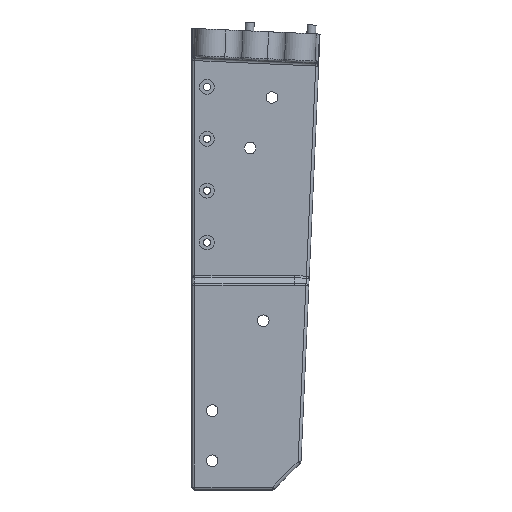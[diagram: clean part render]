
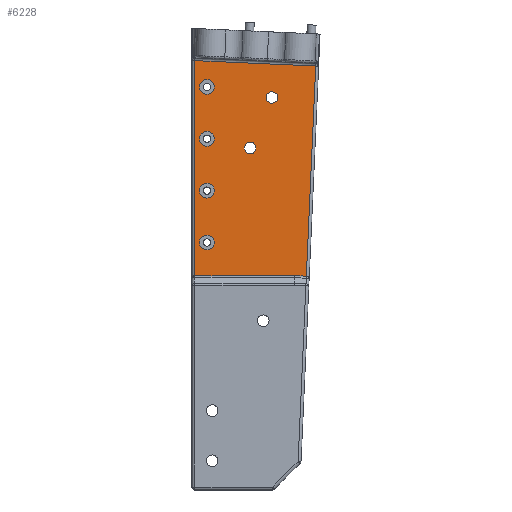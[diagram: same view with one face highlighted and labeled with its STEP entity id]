
A CAD part, left-side view. The second image highlights one B-rep face of the part: STEP entity #6228.
In plain terms, the highlighted planar face has unit normal (-1, 0, 0).
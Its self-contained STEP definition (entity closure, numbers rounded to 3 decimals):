
#161=ELLIPSE('',#6764,2.83,2.);
#335=LINE('',#9959,#885);
#356=LINE('',#10603,#906);
#358=LINE('',#10630,#908);
#368=LINE('',#10674,#918);
#369=LINE('',#10676,#919);
#885=VECTOR('',#7695,10.);
#906=VECTOR('',#7892,10.);
#908=VECTOR('',#7904,10.);
#918=VECTOR('',#7932,10.);
#919=VECTOR('',#7935,10.);
#1436=FACE_BOUND('',#2027,.T.);
#1437=FACE_BOUND('',#2028,.T.);
#1438=FACE_BOUND('',#2029,.T.);
#1439=FACE_BOUND('',#2030,.T.);
#1440=FACE_BOUND('',#2031,.T.);
#1441=FACE_BOUND('',#2032,.T.);
#1622=FACE_OUTER_BOUND('',#2026,.T.);
#2026=EDGE_LOOP('',(#4883,#4884,#4885,#4886,#4887,#4888));
#2027=EDGE_LOOP('',(#4889,#4890));
#2028=EDGE_LOOP('',(#4891,#4892));
#2029=EDGE_LOOP('',(#4893,#4894));
#2030=EDGE_LOOP('',(#4895,#4896));
#2031=EDGE_LOOP('',(#4897,#4898));
#2032=EDGE_LOOP('',(#4899));
#2284=CIRCLE('',#6493,2.54);
#2285=CIRCLE('',#6494,2.54);
#2289=CIRCLE('',#6500,2.54);
#2290=CIRCLE('',#6501,2.54);
#2294=CIRCLE('',#6507,2.54);
#2295=CIRCLE('',#6508,2.54);
#2299=CIRCLE('',#6514,2.54);
#2300=CIRCLE('',#6515,2.54);
#2474=CIRCLE('',#6821,2.);
#2475=CIRCLE('',#6822,2.);
#2476=CIRCLE('',#6823,2.);
#2621=VERTEX_POINT('',#9115);
#2622=VERTEX_POINT('',#9117);
#2626=VERTEX_POINT('',#9128);
#2627=VERTEX_POINT('',#9130);
#2631=VERTEX_POINT('',#9141);
#2632=VERTEX_POINT('',#9143);
#2636=VERTEX_POINT('',#9154);
#2637=VERTEX_POINT('',#9156);
#2790=VERTEX_POINT('',#9945);
#2794=VERTEX_POINT('',#9957);
#2872=VERTEX_POINT('',#10594);
#2875=VERTEX_POINT('',#10601);
#2877=VERTEX_POINT('',#10622);
#2879=VERTEX_POINT('',#10628);
#2905=VERTEX_POINT('',#10844);
#2906=VERTEX_POINT('',#10845);
#2907=VERTEX_POINT('',#10848);
#3219=EDGE_CURVE('',#2622,#2621,#2284,.T.);
#3220=EDGE_CURVE('',#2621,#2622,#2285,.T.);
#3225=EDGE_CURVE('',#2627,#2626,#2289,.T.);
#3226=EDGE_CURVE('',#2626,#2627,#2290,.T.);
#3231=EDGE_CURVE('',#2632,#2631,#2294,.T.);
#3232=EDGE_CURVE('',#2631,#2632,#2295,.T.);
#3237=EDGE_CURVE('',#2637,#2636,#2299,.T.);
#3238=EDGE_CURVE('',#2636,#2637,#2300,.T.);
#3453=EDGE_CURVE('',#2794,#2790,#335,.T.);
#3564=EDGE_CURVE('',#2875,#2872,#356,.T.);
#3567=EDGE_CURVE('',#2877,#2875,#161,.T.);
#3570=EDGE_CURVE('',#2879,#2877,#358,.T.);
#3584=EDGE_CURVE('',#2872,#2794,#368,.T.);
#3585=EDGE_CURVE('',#2790,#2879,#369,.T.);
#3637=EDGE_CURVE('',#2905,#2906,#2474,.T.);
#3638=EDGE_CURVE('',#2906,#2905,#2475,.T.);
#3639=EDGE_CURVE('',#2907,#2907,#2476,.T.);
#4883=ORIENTED_EDGE('',*,*,#3453,.F.);
#4884=ORIENTED_EDGE('',*,*,#3584,.F.);
#4885=ORIENTED_EDGE('',*,*,#3564,.F.);
#4886=ORIENTED_EDGE('',*,*,#3567,.F.);
#4887=ORIENTED_EDGE('',*,*,#3570,.F.);
#4888=ORIENTED_EDGE('',*,*,#3585,.F.);
#4889=ORIENTED_EDGE('',*,*,#3219,.T.);
#4890=ORIENTED_EDGE('',*,*,#3220,.T.);
#4891=ORIENTED_EDGE('',*,*,#3225,.T.);
#4892=ORIENTED_EDGE('',*,*,#3226,.T.);
#4893=ORIENTED_EDGE('',*,*,#3231,.T.);
#4894=ORIENTED_EDGE('',*,*,#3232,.T.);
#4895=ORIENTED_EDGE('',*,*,#3237,.T.);
#4896=ORIENTED_EDGE('',*,*,#3238,.T.);
#4897=ORIENTED_EDGE('',*,*,#3637,.T.);
#4898=ORIENTED_EDGE('',*,*,#3638,.T.);
#4899=ORIENTED_EDGE('',*,*,#3639,.T.);
#5942=PLANE('',#6820);
#6228=ADVANCED_FACE('',(#1622,#1436,#1437,#1438,#1439,#1440,#1441),#5942,
 .F.);
#6493=AXIS2_PLACEMENT_3D('',#9118,#7232,#7233);
#6494=AXIS2_PLACEMENT_3D('',#9119,#7234,#7235);
#6500=AXIS2_PLACEMENT_3D('',#9131,#7247,#7248);
#6501=AXIS2_PLACEMENT_3D('',#9132,#7249,#7250);
#6507=AXIS2_PLACEMENT_3D('',#9144,#7262,#7263);
#6508=AXIS2_PLACEMENT_3D('',#9145,#7264,#7265);
#6514=AXIS2_PLACEMENT_3D('',#9157,#7277,#7278);
#6515=AXIS2_PLACEMENT_3D('',#9158,#7279,#7280);
#6764=AXIS2_PLACEMENT_3D('',#10624,#7896,#7897);
#6820=AXIS2_PLACEMENT_3D('',#10843,#8059,#8060);
#6821=AXIS2_PLACEMENT_3D('',#10846,#8061,#8062);
#6822=AXIS2_PLACEMENT_3D('',#10847,#8063,#8064);
#6823=AXIS2_PLACEMENT_3D('',#10849,#8065,#8066);
#7232=DIRECTION('center_axis',(1.,0.,0.));
#7233=DIRECTION('ref_axis',(0.,0.,-1.));
#7234=DIRECTION('center_axis',(1.,0.,0.));
#7235=DIRECTION('ref_axis',(0.,0.,-1.));
#7247=DIRECTION('center_axis',(1.,0.,0.));
#7248=DIRECTION('ref_axis',(0.,0.,-1.));
#7249=DIRECTION('center_axis',(1.,0.,0.));
#7250=DIRECTION('ref_axis',(0.,0.,-1.));
#7262=DIRECTION('center_axis',(1.,0.,0.));
#7263=DIRECTION('ref_axis',(0.,0.,-1.));
#7264=DIRECTION('center_axis',(1.,0.,0.));
#7265=DIRECTION('ref_axis',(0.,0.,-1.));
#7277=DIRECTION('center_axis',(1.,0.,0.));
#7278=DIRECTION('ref_axis',(0.,0.,-1.));
#7279=DIRECTION('center_axis',(1.,0.,0.));
#7280=DIRECTION('ref_axis',(0.,0.,-1.));
#7695=DIRECTION('',(0.,-0.999,-0.044));
#7892=DIRECTION('',(0.,1.,0.));
#7896=DIRECTION('center_axis',(-1.,0.,0.));
#7897=DIRECTION('ref_axis',(0.,-0.044,0.999));
#7904=DIRECTION('',(0.,0.999,0.044));
#7932=DIRECTION('',(0.,0.,1.));
#7935=DIRECTION('',(0.,0.044,-0.999));
#8059=DIRECTION('center_axis',(1.,0.,0.));
#8060=DIRECTION('ref_axis',(0.,0.,-1.));
#8061=DIRECTION('center_axis',(1.,0.,0.));
#8062=DIRECTION('ref_axis',(0.,0.,1.));
#8063=DIRECTION('center_axis',(1.,0.,0.));
#8064=DIRECTION('ref_axis',(0.,0.,1.));
#8065=DIRECTION('center_axis',(1.,0.,0.));
#8066=DIRECTION('ref_axis',(0.,0.,1.));
#9115=CARTESIAN_POINT('',(-27.1,-5.186,105.126));
#9117=CARTESIAN_POINT('',(-27.1,-5.186,100.046));
#9118=CARTESIAN_POINT('Origin',(-27.1,-5.186,102.586));
#9119=CARTESIAN_POINT('Origin',(-27.1,-5.186,102.586));
#9128=CARTESIAN_POINT('',(-27.1,-5.186,122.906));
#9130=CARTESIAN_POINT('',(-27.1,-5.186,117.826));
#9131=CARTESIAN_POINT('Origin',(-27.1,-5.186,120.366));
#9132=CARTESIAN_POINT('Origin',(-27.1,-5.186,120.366));
#9141=CARTESIAN_POINT('',(-27.1,-5.186,87.346));
#9143=CARTESIAN_POINT('',(-27.1,-5.186,82.266));
#9144=CARTESIAN_POINT('Origin',(-27.1,-5.186,84.806));
#9145=CARTESIAN_POINT('Origin',(-27.1,-5.186,84.806));
#9154=CARTESIAN_POINT('',(-27.1,-5.186,140.686));
#9156=CARTESIAN_POINT('',(-27.1,-5.186,135.606));
#9157=CARTESIAN_POINT('Origin',(-27.1,-5.186,138.146));
#9158=CARTESIAN_POINT('Origin',(-27.1,-5.186,138.146));
#9945=CARTESIAN_POINT('',(-27.1,-42.475,145.293));
#9957=CARTESIAN_POINT('',(-27.1,-1.086,147.136));
#9959=CARTESIAN_POINT('',(-27.1,-22.548,146.181));
#10594=CARTESIAN_POINT('',(-27.1,-1.086,73.456));
#10601=CARTESIAN_POINT('',(-27.1,-35.224,73.456));
#10603=CARTESIAN_POINT('',(-27.1,-11.034,73.456));
#10622=CARTESIAN_POINT('',(-27.1,-35.287,73.454));
#10624=CARTESIAN_POINT('Origin',(-27.1,-35.161,70.627));
#10628=CARTESIAN_POINT('',(-27.1,-39.267,73.277));
#10630=CARTESIAN_POINT('',(-27.1,-27.812,73.787));
#10674=CARTESIAN_POINT('',(-27.1,-1.086,55.823));
#10676=CARTESIAN_POINT('',(-27.1,-39.739,83.86));
#10843=CARTESIAN_POINT('Origin',(-27.1,-22.024,111.646));
#10844=CARTESIAN_POINT('',(-27.1,-20.,115.2));
#10845=CARTESIAN_POINT('',(-27.1,-20.,119.2));
#10846=CARTESIAN_POINT('Origin',(-27.1,-20.,117.2));
#10847=CARTESIAN_POINT('Origin',(-27.1,-20.,117.2));
#10848=CARTESIAN_POINT('',(-27.1,-27.5,132.5));
#10849=CARTESIAN_POINT('Origin',(-27.1,-27.5,134.5));
